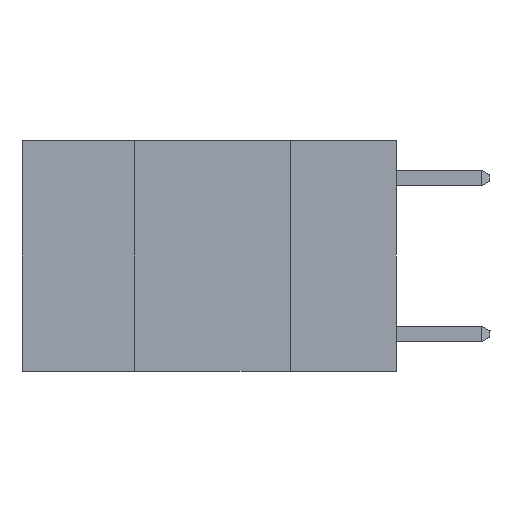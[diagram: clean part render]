
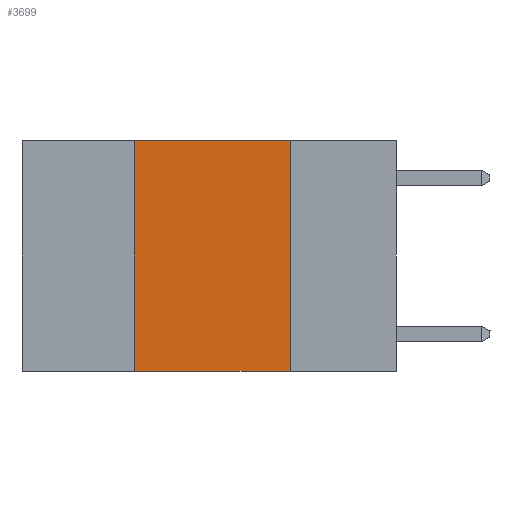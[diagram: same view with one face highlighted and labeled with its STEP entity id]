
A CAD part, left-side view. The second image highlights one B-rep face of the part: STEP entity #3699.
In plain terms, the highlighted planar face has unit normal (-1, 0, 0).
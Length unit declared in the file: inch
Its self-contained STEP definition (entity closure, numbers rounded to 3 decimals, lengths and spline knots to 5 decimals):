
#542 = CARTESIAN_POINT ( 'NONE',  ( 0., 0.42, -0.37 ) ) ;
#564 = VECTOR ( 'NONE', #12302, 39.37008 ) ;
#807 = CARTESIAN_POINT ( 'NONE',  ( 0., 0.42, 0. ) ) ;
#2221 = CARTESIAN_POINT ( 'NONE',  ( 0., 0.17, -0.37 ) ) ;
#2226 = DIRECTION ( 'NONE',  ( 0., 0., 1. ) ) ;
#2403 = ORIENTED_EDGE ( 'NONE', *, *, #11035, .T. ) ;
#2788 = DIRECTION ( 'NONE',  ( 0., 0., -1. ) ) ;
#2898 = DIRECTION ( 'NONE',  ( 1., 0., 0. ) ) ;
#2915 = CARTESIAN_POINT ( 'NONE',  ( 0., 0.6, 0. ) ) ;
#2929 = PLANE ( 'NONE',  #7399 ) ;
#3285 = LINE ( 'NONE', #8376, #5954 ) ;
#3699 = ADVANCED_FACE ( 'NONE', ( #11670 ), #2929, .F. ) ;
#4035 = EDGE_CURVE ( 'NONE', #11222, #10086, #12554, .T. ) ;
#4846 = VERTEX_POINT ( 'NONE', #542 ) ;
#5034 = LINE ( 'NONE', #9300, #9884 ) ;
#5858 = VERTEX_POINT ( 'NONE', #2221 ) ;
#5954 = VECTOR ( 'NONE', #9342, 39.37008 ) ;
#7399 = AXIS2_PLACEMENT_3D ( 'NONE', #2915, #2898, #2788 ) ;
#8113 = CARTESIAN_POINT ( 'NONE',  ( 0., 0.42, 0. ) ) ;
#8376 = CARTESIAN_POINT ( 'NONE',  ( 0., 0.6, -0.37 ) ) ;
#8581 = LINE ( 'NONE', #8113, #9193 ) ;
#8878 = EDGE_CURVE ( 'NONE', #4846, #11222, #8581, .T. ) ;
#9193 = VECTOR ( 'NONE', #2226, 39.37008 ) ;
#9298 = ORIENTED_EDGE ( 'NONE', *, *, #4035, .F. ) ;
#9300 = CARTESIAN_POINT ( 'NONE',  ( 0., 0.17, 0. ) ) ;
#9342 = DIRECTION ( 'NONE',  ( 0., -1., 0. ) ) ;
#9591 = ORIENTED_EDGE ( 'NONE', *, *, #8878, .F. ) ;
#9884 = VECTOR ( 'NONE', #10238, 39.37008 ) ;
#10086 = VERTEX_POINT ( 'NONE', #10845 ) ;
#10229 = EDGE_CURVE ( 'NONE', #10086, #5858, #5034, .T. ) ;
#10238 = DIRECTION ( 'NONE',  ( 0., 0., -1. ) ) ;
#10495 = EDGE_LOOP ( 'NONE', ( #11527, #9298, #9591, #2403 ) ) ;
#10845 = CARTESIAN_POINT ( 'NONE',  ( 0., 0.17, 0. ) ) ;
#11035 = EDGE_CURVE ( 'NONE', #4846, #5858, #3285, .T. ) ;
#11222 = VERTEX_POINT ( 'NONE', #807 ) ;
#11527 = ORIENTED_EDGE ( 'NONE', *, *, #10229, .F. ) ;
#11670 = FACE_OUTER_BOUND ( 'NONE', #10495, .T. ) ;
#12154 = CARTESIAN_POINT ( 'NONE',  ( 0., 0.6, 0. ) ) ;
#12302 = DIRECTION ( 'NONE',  ( 0., -1., 0. ) ) ;
#12554 = LINE ( 'NONE', #12154, #564 ) ;
